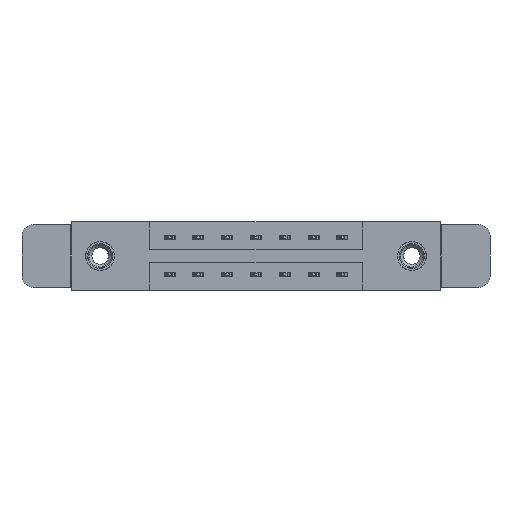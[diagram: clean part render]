
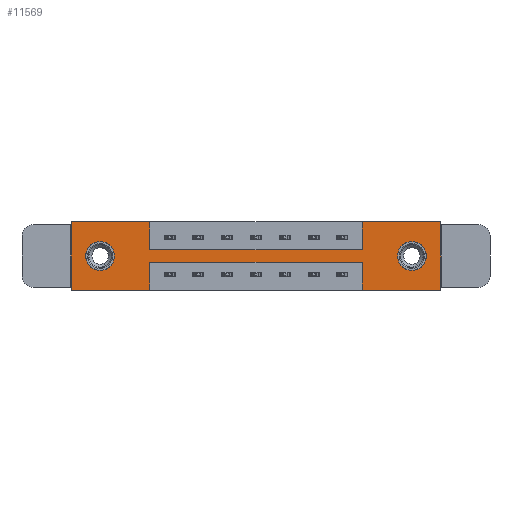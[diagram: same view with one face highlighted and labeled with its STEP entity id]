
A CAD part, front view. The second image highlights one B-rep face of the part: STEP entity #11569.
In plain terms, the highlighted planar face has unit normal (0, -1, 0).
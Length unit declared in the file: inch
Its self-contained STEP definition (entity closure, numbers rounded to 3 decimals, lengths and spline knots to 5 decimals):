
#54 = CARTESIAN_POINT ( 'NONE',  ( 1.998, 0., 0. ) ) ;
#72 = VERTEX_POINT ( 'NONE', #8864 ) ;
#87 = CIRCLE ( 'NONE', #476, 0.078 ) ;
#100 = DIRECTION ( 'NONE',  ( 0., 0., -1. ) ) ;
#212 = EDGE_LOOP ( 'NONE', ( #802, #713, #2867, #5147, #9229, #7950, #2557, #727, #5863, #12335, #7683, #4404 ) ) ;
#359 = LINE ( 'NONE', #7022, #5733 ) ;
#392 = ORIENTED_EDGE ( 'NONE', *, *, #1334, .T. ) ;
#476 = AXIS2_PLACEMENT_3D ( 'NONE', #7887, #6940, #1088 ) ;
#713 = ORIENTED_EDGE ( 'NONE', *, *, #12536, .F. ) ;
#727 = ORIENTED_EDGE ( 'NONE', *, *, #7369, .F. ) ;
#753 = VERTEX_POINT ( 'NONE', #9056 ) ;
#802 = ORIENTED_EDGE ( 'NONE', *, *, #10000, .F. ) ;
#930 = LINE ( 'NONE', #7567, #9903 ) ;
#1024 = FACE_BOUND ( 'NONE', #7226, .T. ) ;
#1025 = CARTESIAN_POINT ( 'NONE',  ( 0.155, 0., -0.185 ) ) ;
#1088 = DIRECTION ( 'NONE',  ( 0., 0., -1. ) ) ;
#1188 = DIRECTION ( 'NONE',  ( 0., 0., -1. ) ) ;
#1193 = CARTESIAN_POINT ( 'NONE',  ( 1.998, 0., 0. ) ) ;
#1334 = EDGE_CURVE ( 'NONE', #3999, #11721, #9018, .T. ) ;
#1713 = LINE ( 'NONE', #54, #5702 ) ;
#1881 = CARTESIAN_POINT ( 'NONE',  ( 0., 0., 0. ) ) ;
#1883 = LINE ( 'NONE', #1881, #5565 ) ;
#1907 = VERTEX_POINT ( 'NONE', #9055 ) ;
#2149 = VECTOR ( 'NONE', #9964, 39.37008 ) ;
#2204 = CARTESIAN_POINT ( 'NONE',  ( 0.425, 0., -0.37 ) ) ;
#2275 = LINE ( 'NONE', #11273, #4731 ) ;
#2281 = CARTESIAN_POINT ( 'NONE',  ( 0.425, 0., -0.15 ) ) ;
#2398 = EDGE_CURVE ( 'NONE', #3169, #9071, #87, .T. ) ;
#2428 = VERTEX_POINT ( 'NONE', #4129 ) ;
#2557 = ORIENTED_EDGE ( 'NONE', *, *, #8843, .F. ) ;
#2626 = CARTESIAN_POINT ( 'NONE',  ( 0., 0., -0.37 ) ) ;
#2750 = EDGE_CURVE ( 'NONE', #11721, #3999, #3326, .T. ) ;
#2843 = VERTEX_POINT ( 'NONE', #1193 ) ;
#2867 = ORIENTED_EDGE ( 'NONE', *, *, #9132, .F. ) ;
#2899 = DIRECTION ( 'NONE',  ( 1., 0., 0. ) ) ;
#2985 = FACE_BOUND ( 'NONE', #10322, .T. ) ;
#3154 = CARTESIAN_POINT ( 'NONE',  ( 1.573, 0., -0.15 ) ) ;
#3169 = VERTEX_POINT ( 'NONE', #9431 ) ;
#3326 = CIRCLE ( 'NONE', #4163, 0.078 ) ;
#3336 = DIRECTION ( 'NONE',  ( 1., 0., 0. ) ) ;
#3454 = CARTESIAN_POINT ( 'NONE',  ( 0.425, 0., -0.22 ) ) ;
#3534 = DIRECTION ( 'NONE',  ( 0., 0., -1. ) ) ;
#3627 = AXIS2_PLACEMENT_3D ( 'NONE', #4826, #9937, #4898 ) ;
#3959 = DIRECTION ( 'NONE',  ( 0., 1., 0. ) ) ;
#3999 = VERTEX_POINT ( 'NONE', #7289 ) ;
#4045 = LINE ( 'NONE', #3454, #11660 ) ;
#4129 = CARTESIAN_POINT ( 'NONE',  ( 0.425, 0., -0.22 ) ) ;
#4163 = AXIS2_PLACEMENT_3D ( 'NONE', #1025, #3959, #4941 ) ;
#4174 = DIRECTION ( 'NONE',  ( -1., 0., 0. ) ) ;
#4404 = ORIENTED_EDGE ( 'NONE', *, *, #9602, .F. ) ;
#4544 = FACE_OUTER_BOUND ( 'NONE', #212, .T. ) ;
#4731 = VECTOR ( 'NONE', #3336, 39.37008 ) ;
#4762 = LINE ( 'NONE', #2281, #2149 ) ;
#4826 = CARTESIAN_POINT ( 'NONE',  ( 1.843, 0., -0.185 ) ) ;
#4898 = DIRECTION ( 'NONE',  ( 0., 0., -1. ) ) ;
#4941 = DIRECTION ( 'NONE',  ( 0., 0., 1. ) ) ;
#5110 = CARTESIAN_POINT ( 'NONE',  ( 1.998, 0., -0.37 ) ) ;
#5142 = VERTEX_POINT ( 'NONE', #5110 ) ;
#5147 = ORIENTED_EDGE ( 'NONE', *, *, #10051, .F. ) ;
#5220 = AXIS2_PLACEMENT_3D ( 'NONE', #11252, #10452, #9326 ) ;
#5372 = VERTEX_POINT ( 'NONE', #9416 ) ;
#5422 = CARTESIAN_POINT ( 'NONE',  ( 0., 0., -0.37 ) ) ;
#5565 = VECTOR ( 'NONE', #2899, 39.37008 ) ;
#5702 = VECTOR ( 'NONE', #100, 39.37008 ) ;
#5733 = VECTOR ( 'NONE', #7100, 39.37008 ) ;
#5863 = ORIENTED_EDGE ( 'NONE', *, *, #7682, .F. ) ;
#5880 = CARTESIAN_POINT ( 'NONE',  ( 0., 0., 0. ) ) ;
#6029 = EDGE_CURVE ( 'NONE', #72, #753, #1883, .T. ) ;
#6099 = CARTESIAN_POINT ( 'NONE',  ( 0.155, 0., -0.107 ) ) ;
#6110 = VECTOR ( 'NONE', #1188, 39.37008 ) ;
#6253 = VECTOR ( 'NONE', #7027, 39.37008 ) ;
#6333 = DIRECTION ( 'NONE',  ( -1., 0., 0. ) ) ;
#6400 = CARTESIAN_POINT ( 'NONE',  ( 1.843, 0., -0.263 ) ) ;
#6412 = LINE ( 'NONE', #7985, #9129 ) ;
#6703 = CARTESIAN_POINT ( 'NONE',  ( 1.573, 0., -0.22 ) ) ;
#6707 = EDGE_CURVE ( 'NONE', #2843, #5142, #1713, .T. ) ;
#6911 = ORIENTED_EDGE ( 'NONE', *, *, #2750, .T. ) ;
#6940 = DIRECTION ( 'NONE',  ( 0., 1., 0. ) ) ;
#7022 = CARTESIAN_POINT ( 'NONE',  ( 1.573, 0., 0. ) ) ;
#7027 = DIRECTION ( 'NONE',  ( 0., 0., 1. ) ) ;
#7100 = DIRECTION ( 'NONE',  ( 0., 0., 1. ) ) ;
#7126 = VERTEX_POINT ( 'NONE', #6703 ) ;
#7226 = EDGE_LOOP ( 'NONE', ( #6911, #392 ) ) ;
#7289 = CARTESIAN_POINT ( 'NONE',  ( 0.155, 0., -0.263 ) ) ;
#7369 = EDGE_CURVE ( 'NONE', #9320, #9894, #4762, .T. ) ;
#7474 = PLANE ( 'NONE',  #8190 ) ;
#7567 = CARTESIAN_POINT ( 'NONE',  ( 1.573, 0., -0.37 ) ) ;
#7625 = CARTESIAN_POINT ( 'NONE',  ( 0.425, 0., 0. ) ) ;
#7682 = EDGE_CURVE ( 'NONE', #753, #9320, #8240, .T. ) ;
#7683 = ORIENTED_EDGE ( 'NONE', *, *, #10476, .F. ) ;
#7887 = CARTESIAN_POINT ( 'NONE',  ( 1.843, 0., -0.185 ) ) ;
#7913 = VECTOR ( 'NONE', #3534, 39.37008 ) ;
#7916 = ORIENTED_EDGE ( 'NONE', *, *, #8715, .T. ) ;
#7950 = ORIENTED_EDGE ( 'NONE', *, *, #8420, .F. ) ;
#7979 = CARTESIAN_POINT ( 'NONE',  ( 1.573, 0., 0. ) ) ;
#7985 = CARTESIAN_POINT ( 'NONE',  ( 0., 0., -0.37 ) ) ;
#8001 = CARTESIAN_POINT ( 'NONE',  ( 0.425, 0., -0.15 ) ) ;
#8119 = VERTEX_POINT ( 'NONE', #11782 ) ;
#8190 = AXIS2_PLACEMENT_3D ( 'NONE', #2626, #11410, #9476 ) ;
#8218 = LINE ( 'NONE', #2204, #6110 ) ;
#8240 = LINE ( 'NONE', #7625, #7913 ) ;
#8420 = EDGE_CURVE ( 'NONE', #10130, #2843, #2275, .T. ) ;
#8715 = EDGE_CURVE ( 'NONE', #9071, #3169, #9870, .T. ) ;
#8843 = EDGE_CURVE ( 'NONE', #9894, #10130, #359, .T. ) ;
#8864 = CARTESIAN_POINT ( 'NONE',  ( 0., 0., 0. ) ) ;
#9018 = CIRCLE ( 'NONE', #5220, 0.078 ) ;
#9055 = CARTESIAN_POINT ( 'NONE',  ( 0.425, 0., -0.37 ) ) ;
#9056 = CARTESIAN_POINT ( 'NONE',  ( 0.425, 0., 0. ) ) ;
#9071 = VERTEX_POINT ( 'NONE', #6400 ) ;
#9129 = VECTOR ( 'NONE', #4174, 39.37008 ) ;
#9132 = EDGE_CURVE ( 'NONE', #5372, #7126, #930, .T. ) ;
#9229 = ORIENTED_EDGE ( 'NONE', *, *, #6707, .F. ) ;
#9265 = LINE ( 'NONE', #5880, #6253 ) ;
#9320 = VERTEX_POINT ( 'NONE', #8001 ) ;
#9326 = DIRECTION ( 'NONE',  ( 0., 0., 1. ) ) ;
#9416 = CARTESIAN_POINT ( 'NONE',  ( 1.573, 0., -0.37 ) ) ;
#9431 = CARTESIAN_POINT ( 'NONE',  ( 1.843, 0., -0.107 ) ) ;
#9476 = DIRECTION ( 'NONE',  ( 0., 0., -1. ) ) ;
#9602 = EDGE_CURVE ( 'NONE', #1907, #8119, #6412, .T. ) ;
#9870 = CIRCLE ( 'NONE', #3627, 0.078 ) ;
#9894 = VERTEX_POINT ( 'NONE', #3154 ) ;
#9903 = VECTOR ( 'NONE', #10468, 39.37008 ) ;
#9937 = DIRECTION ( 'NONE',  ( 0., 1., 0. ) ) ;
#9964 = DIRECTION ( 'NONE',  ( 1., 0., 0. ) ) ;
#10000 = EDGE_CURVE ( 'NONE', #2428, #1907, #8218, .T. ) ;
#10051 = EDGE_CURVE ( 'NONE', #5142, #5372, #12036, .T. ) ;
#10130 = VERTEX_POINT ( 'NONE', #7979 ) ;
#10322 = EDGE_LOOP ( 'NONE', ( #11624, #7916 ) ) ;
#10452 = DIRECTION ( 'NONE',  ( 0., 1., 0. ) ) ;
#10468 = DIRECTION ( 'NONE',  ( 0., 0., 1. ) ) ;
#10476 = EDGE_CURVE ( 'NONE', #8119, #72, #9265, .T. ) ;
#11252 = CARTESIAN_POINT ( 'NONE',  ( 0.155, 0., -0.185 ) ) ;
#11273 = CARTESIAN_POINT ( 'NONE',  ( 0., 0., 0. ) ) ;
#11410 = DIRECTION ( 'NONE',  ( 0., -1., 0. ) ) ;
#11569 = ADVANCED_FACE ( 'NONE', ( #2985, #1024, #4544 ), #7474, .T. ) ;
#11624 = ORIENTED_EDGE ( 'NONE', *, *, #2398, .T. ) ;
#11660 = VECTOR ( 'NONE', #6333, 39.37008 ) ;
#11717 = VECTOR ( 'NONE', #12385, 39.37008 ) ;
#11721 = VERTEX_POINT ( 'NONE', #6099 ) ;
#11782 = CARTESIAN_POINT ( 'NONE',  ( 0., 0., -0.37 ) ) ;
#12036 = LINE ( 'NONE', #5422, #11717 ) ;
#12335 = ORIENTED_EDGE ( 'NONE', *, *, #6029, .F. ) ;
#12385 = DIRECTION ( 'NONE',  ( -1., 0., 0. ) ) ;
#12536 = EDGE_CURVE ( 'NONE', #7126, #2428, #4045, .T. ) ;
